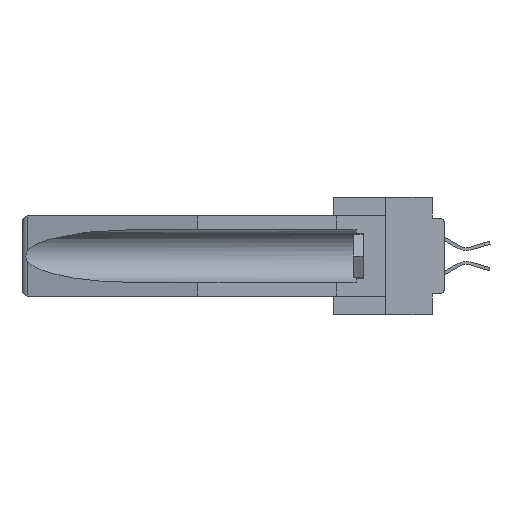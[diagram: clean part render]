
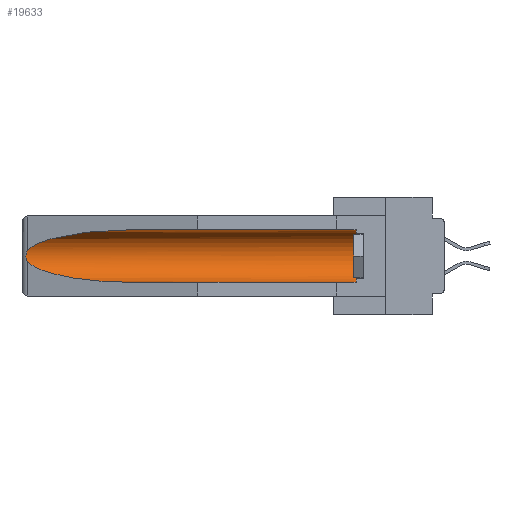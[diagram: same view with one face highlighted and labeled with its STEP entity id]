
A CAD part, left-side view. The second image highlights one B-rep face of the part: STEP entity #19633.
In plain terms, the highlighted cylindrical face has radius 2.857 mm (diameter 5.715 mm), a partial arc.
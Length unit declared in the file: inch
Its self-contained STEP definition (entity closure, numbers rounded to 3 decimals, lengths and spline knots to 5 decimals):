
#747 = CARTESIAN_POINT ( 'NONE',  ( 0.26597, 1.5296, -0.19026 ) ) ;
#2839 = LINE ( 'NONE', #14224, #33679 ) ;
#2891 = DIRECTION ( 'NONE',  ( 0., 1., 0. ) ) ;
#4123 = ORIENTED_EDGE ( 'NONE', *, *, #24093, .T. ) ;
#4293 = ORIENTED_EDGE ( 'NONE', *, *, #33725, .T. ) ;
#4349 = CARTESIAN_POINT ( 'NONE',  ( 0.25451, 1.48313, -0.09465 ) ) ;
#4562 = EDGE_LOOP ( 'NONE', ( #29610, #11325, #4123, #13850, #4293, #20911 ) ) ;
#5809 = CIRCLE ( 'NONE', #8795, 0.1125 ) ;
#6122 = VERTEX_POINT ( 'NONE', #22963 ) ;
#7084 = EDGE_CURVE ( 'NONE', #33652, #15548, #10707, .T. ) ;
#8053 = DIRECTION ( 'NONE',  ( 0., 1., 0. ) ) ;
#8601 = CARTESIAN_POINT ( 'NONE',  ( 0.155, 1.07973, -0.284 ) ) ;
#8795 = AXIS2_PLACEMENT_3D ( 'NONE', #11369, #31523, #25911 ) ;
#9555 = EDGE_CURVE ( 'NONE', #6122, #23671, #23130, .T. ) ;
#10131 = CARTESIAN_POINT ( 'NONE',  ( 0.21114, 1.30732, -0.059 ) ) ;
#10281 =( BOUNDED_CURVE ( )  B_SPLINE_CURVE ( 3, ( #36414, #10131, #4349, #22255 ),
 .UNSPECIFIED., .F., .T. ) 
 B_SPLINE_CURVE_WITH_KNOTS ( ( 4, 4 ),
 ( 4.71239, 6.08839 ),
 .UNSPECIFIED. ) 
 CURVE ( )  GEOMETRIC_REPRESENTATION_ITEM ( )  RATIONAL_B_SPLINE_CURVE ( ( 1., 0.848, 0.848, 1. ) ) 
 REPRESENTATION_ITEM ( '' )  );
#10707 = B_SPLINE_CURVE_WITH_KNOTS ( 'NONE', 3,
 ( #23875, #31718, #29292, #34716, #14548, #17948, #20351, #25930, #747, #12122 ),
 .UNSPECIFIED., .F., .F.,
 ( 4, 2, 2, 2, 4 ),
 ( 0., 0.00029, 0.00058, 0.00087, 0.00117 ),
 .UNSPECIFIED. ) ;
#11042 = CARTESIAN_POINT ( 'NONE',  ( 0.155, 1.07973, -0.059 ) ) ;
#11325 = ORIENTED_EDGE ( 'NONE', *, *, #7084, .T. ) ;
#11369 = CARTESIAN_POINT ( 'NONE',  ( 0.155, 0.126, -0.1715 ) ) ;
#11977 = VERTEX_POINT ( 'NONE', #11042 ) ;
#12052 = AXIS2_PLACEMENT_3D ( 'NONE', #28624, #2891, #14267 ) ;
#12122 = CARTESIAN_POINT ( 'NONE',  ( 0.26537, 1.52718, -0.19328 ) ) ;
#12271 = EDGE_CURVE ( 'NONE', #27729, #11977, #2839, .T. ) ;
#13850 = ORIENTED_EDGE ( 'NONE', *, *, #9555, .F. ) ;
#14224 = CARTESIAN_POINT ( 'NONE',  ( 0.155, -0.30754, -0.059 ) ) ;
#14267 = DIRECTION ( 'NONE',  ( 0., 0., 1. ) ) ;
#14548 = CARTESIAN_POINT ( 'NONE',  ( 0.2675, 1.53308, -0.16763 ) ) ;
#14601 = CARTESIAN_POINT ( 'NONE',  ( 0.155, 1.07973, -0.284 ) ) ;
#15548 = VERTEX_POINT ( 'NONE', #21633 ) ;
#17948 = CARTESIAN_POINT ( 'NONE',  ( 0.2675, 1.53308, -0.17534 ) ) ;
#19027 = FACE_OUTER_BOUND ( 'NONE', #4562, .T. ) ;
#19237 = CARTESIAN_POINT ( 'NONE',  ( 0.26537, 1.52718, -0.14972 ) ) ;
#19633 = ADVANCED_FACE ( 'NONE', ( #19027 ), #31791, .F. ) ;
#20351 = CARTESIAN_POINT ( 'NONE',  ( 0.2673, 1.53269, -0.17917 ) ) ;
#20911 = ORIENTED_EDGE ( 'NONE', *, *, #12271, .T. ) ;
#21633 = CARTESIAN_POINT ( 'NONE',  ( 0.26537, 1.52718, -0.19328 ) ) ;
#22255 = CARTESIAN_POINT ( 'NONE',  ( 0.26537, 1.52718, -0.14972 ) ) ;
#22963 = CARTESIAN_POINT ( 'NONE',  ( 0.155, 0.126, -0.284 ) ) ;
#23130 = LINE ( 'NONE', #33625, #35572 ) ;
#23671 = VERTEX_POINT ( 'NONE', #14601 ) ;
#23875 = CARTESIAN_POINT ( 'NONE',  ( 0.26537, 1.52718, -0.14972 ) ) ;
#24093 = EDGE_CURVE ( 'NONE', #15548, #23671, #30779, .T. ) ;
#25228 = EDGE_CURVE ( 'NONE', #11977, #33652, #10281, .T. ) ;
#25911 = DIRECTION ( 'NONE',  ( 0., 0., 1. ) ) ;
#25930 = CARTESIAN_POINT ( 'NONE',  ( 0.26655, 1.53094, -0.18657 ) ) ;
#27729 = VERTEX_POINT ( 'NONE', #27988 ) ;
#27988 = CARTESIAN_POINT ( 'NONE',  ( 0.155, 0.126, -0.059 ) ) ;
#28198 = CARTESIAN_POINT ( 'NONE',  ( 0.26537, 1.52718, -0.19328 ) ) ;
#28624 = CARTESIAN_POINT ( 'NONE',  ( 0.155, -0.30754, -0.1715 ) ) ;
#29292 = CARTESIAN_POINT ( 'NONE',  ( 0.26654, 1.53092, -0.15636 ) ) ;
#29610 = ORIENTED_EDGE ( 'NONE', *, *, #25228, .T. ) ;
#30779 =( BOUNDED_CURVE ( )  B_SPLINE_CURVE ( 3, ( #28198, #31370, #36407, #8601 ),
 .UNSPECIFIED., .F., .T. ) 
 B_SPLINE_CURVE_WITH_KNOTS ( ( 4, 4 ),
 ( 0.1948, 1.5708 ),
 .UNSPECIFIED. ) 
 CURVE ( )  GEOMETRIC_REPRESENTATION_ITEM ( )  RATIONAL_B_SPLINE_CURVE ( ( 1., 0.848, 0.848, 1. ) ) 
 REPRESENTATION_ITEM ( '' )  );
#31370 = CARTESIAN_POINT ( 'NONE',  ( 0.25451, 1.48313, -0.24835 ) ) ;
#31523 = DIRECTION ( 'NONE',  ( 0., -1., 0. ) ) ;
#31718 = CARTESIAN_POINT ( 'NONE',  ( 0.26597, 1.52961, -0.15275 ) ) ;
#31791 = CYLINDRICAL_SURFACE ( 'NONE', #12052, 0.1125 ) ;
#33625 = CARTESIAN_POINT ( 'NONE',  ( 0.155, -0.30754, -0.284 ) ) ;
#33652 = VERTEX_POINT ( 'NONE', #19237 ) ;
#33679 = VECTOR ( 'NONE', #35246, 39.37008 ) ;
#33725 = EDGE_CURVE ( 'NONE', #6122, #27729, #5809, .T. ) ;
#34716 = CARTESIAN_POINT ( 'NONE',  ( 0.2673, 1.5327, -0.16383 ) ) ;
#35246 = DIRECTION ( 'NONE',  ( 0., 1., 0. ) ) ;
#35572 = VECTOR ( 'NONE', #8053, 39.37008 ) ;
#36407 = CARTESIAN_POINT ( 'NONE',  ( 0.21114, 1.30732, -0.284 ) ) ;
#36414 = CARTESIAN_POINT ( 'NONE',  ( 0.155, 1.07973, -0.059 ) ) ;
